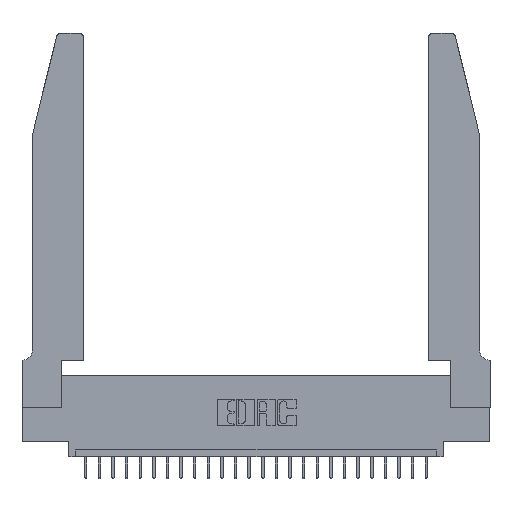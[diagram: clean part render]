
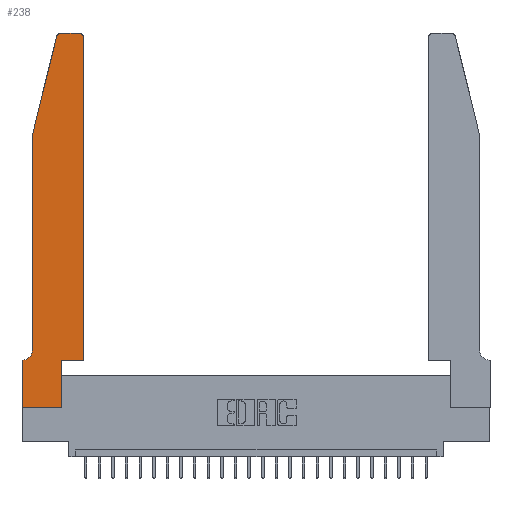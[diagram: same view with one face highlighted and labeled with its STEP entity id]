
A CAD part, top view. The second image highlights one B-rep face of the part: STEP entity #238.
In plain terms, the highlighted planar face has unit normal (0, 0, 1).
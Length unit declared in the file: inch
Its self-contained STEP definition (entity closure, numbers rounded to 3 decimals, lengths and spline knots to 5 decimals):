
#238 = ADVANCED_FACE ( 'NONE', ( #1167 ), #6195, .T. ) ;
#305 = ORIENTED_EDGE ( 'NONE', *, *, #24151, .T. ) ;
#317 = CIRCLE ( 'NONE', #17800, 0.03 ) ;
#383 = CARTESIAN_POINT ( 'NONE',  ( 0., 0., 0.37 ) ) ;
#710 = EDGE_LOOP ( 'NONE', ( #20122, #5138, #15837, #24274, #12912, #5042, #21561, #22669, #1174, #305, #4308, #14873 ) ) ;
#1167 = FACE_OUTER_BOUND ( 'NONE', #710, .T. ) ;
#1174 = ORIENTED_EDGE ( 'NONE', *, *, #11017, .T. ) ;
#1182 = LINE ( 'NONE', #8750, #21146 ) ;
#1298 = EDGE_CURVE ( 'NONE', #10869, #19458, #21773, .T. ) ;
#1369 = DIRECTION ( 'NONE',  ( 0., 1., 0. ) ) ;
#1768 = CARTESIAN_POINT ( 'NONE',  ( 0.284, 2.72, 0.37 ) ) ;
#1846 = EDGE_CURVE ( 'NONE', #4347, #19112, #21419, .T. ) ;
#1937 = EDGE_CURVE ( 'NONE', #4945, #11985, #24655, .T. ) ;
#2071 = CARTESIAN_POINT ( 'NONE',  ( 0.25487, 2.72718, 0.37 ) ) ;
#2384 = CARTESIAN_POINT ( 'NONE',  ( 0.0755, 0.42, 0.37 ) ) ;
#3088 = CARTESIAN_POINT ( 'NONE',  ( 0.4505, 0.35, 0.37 ) ) ;
#3986 = LINE ( 'NONE', #4891, #19770 ) ;
#4308 = ORIENTED_EDGE ( 'NONE', *, *, #10980, .T. ) ;
#4347 = VERTEX_POINT ( 'NONE', #4689 ) ;
#4404 = DIRECTION ( 'NONE',  ( 0., -1., 0. ) ) ;
#4645 = LINE ( 'NONE', #5413, #21703 ) ;
#4689 = CARTESIAN_POINT ( 'NONE',  ( 0., 0.35, 0.37 ) ) ;
#4891 = CARTESIAN_POINT ( 'NONE',  ( 0.2865, 0.35, 0.37 ) ) ;
#4945 = VERTEX_POINT ( 'NONE', #7746 ) ;
#5042 = ORIENTED_EDGE ( 'NONE', *, *, #24692, .T. ) ;
#5044 = CARTESIAN_POINT ( 'NONE',  ( 0.4205, 2.72, 0.37 ) ) ;
#5138 = ORIENTED_EDGE ( 'NONE', *, *, #5745, .T. ) ;
#5211 = DIRECTION ( 'NONE',  ( 1., 0., 0. ) ) ;
#5413 = CARTESIAN_POINT ( 'NONE',  ( 0.4505, 0.35, 0.37 ) ) ;
#5509 = EDGE_CURVE ( 'NONE', #13597, #10869, #10265, .T. ) ;
#5745 = EDGE_CURVE ( 'NONE', #25131, #14039, #317, .T. ) ;
#6195 = PLANE ( 'NONE',  #10839 ) ;
#6304 = LINE ( 'NONE', #13068, #21438 ) ;
#6646 = CARTESIAN_POINT ( 'NONE',  ( 0., 0.35, 0.37 ) ) ;
#6742 = DIRECTION ( 'NONE',  ( -0.239, -0.971, 0. ) ) ;
#6929 = VECTOR ( 'NONE', #10893, 39.37008 ) ;
#7746 = CARTESIAN_POINT ( 'NONE',  ( 0.4505, 2.72, 0.37 ) ) ;
#7828 = CARTESIAN_POINT ( 'NONE',  ( 0.2865, 0.35, 0.37 ) ) ;
#7952 = VECTOR ( 'NONE', #25797, 39.37008 ) ;
#8750 = CARTESIAN_POINT ( 'NONE',  ( 0.0755, 0.35, 0.37 ) ) ;
#8900 = CARTESIAN_POINT ( 'NONE',  ( 0.0755, 2., 0.37 ) ) ;
#8966 = VECTOR ( 'NONE', #4404, 39.37008 ) ;
#10160 = AXIS2_PLACEMENT_3D ( 'NONE', #5044, #19427, #5211 ) ;
#10265 = LINE ( 'NONE', #22926, #8966 ) ;
#10369 = EDGE_CURVE ( 'NONE', #11985, #25131, #21098, .T. ) ;
#10839 = AXIS2_PLACEMENT_3D ( 'NONE', #6646, #12851, #19672 ) ;
#10869 = VERTEX_POINT ( 'NONE', #2384 ) ;
#10893 = DIRECTION ( 'NONE',  ( 0., -1., 0. ) ) ;
#10980 = EDGE_CURVE ( 'NONE', #20373, #4945, #4645, .T. ) ;
#11017 = EDGE_CURVE ( 'NONE', #21164, #11185, #3986, .T. ) ;
#11185 = VERTEX_POINT ( 'NONE', #7828 ) ;
#11408 = VECTOR ( 'NONE', #14041, 39.37008 ) ;
#11512 = CARTESIAN_POINT ( 'NONE',  ( 0.0055, 0.42, 0.37 ) ) ;
#11985 = VERTEX_POINT ( 'NONE', #26577 ) ;
#12652 = CARTESIAN_POINT ( 'NONE',  ( 0.4505, 0.35, 0.37 ) ) ;
#12851 = DIRECTION ( 'NONE',  ( 0., 0., 1. ) ) ;
#12912 = ORIENTED_EDGE ( 'NONE', *, *, #1298, .T. ) ;
#13068 = CARTESIAN_POINT ( 'NONE',  ( 0., 0., 0.37 ) ) ;
#13326 = CARTESIAN_POINT ( 'NONE',  ( 0.0755, 2., 0.37 ) ) ;
#13584 = DIRECTION ( 'NONE',  ( 0., 0., -1. ) ) ;
#13597 = VERTEX_POINT ( 'NONE', #13326 ) ;
#13685 = EDGE_CURVE ( 'NONE', #19112, #21164, #6304, .T. ) ;
#13970 = LINE ( 'NONE', #8900, #21422 ) ;
#14039 = VERTEX_POINT ( 'NONE', #2071 ) ;
#14041 = DIRECTION ( 'NONE',  ( -1., 0., 0. ) ) ;
#14448 = CARTESIAN_POINT ( 'NONE',  ( 0.284, 2.75, 0.37 ) ) ;
#14873 = ORIENTED_EDGE ( 'NONE', *, *, #1937, .T. ) ;
#15837 = ORIENTED_EDGE ( 'NONE', *, *, #25254, .T. ) ;
#16302 = CARTESIAN_POINT ( 'NONE',  ( 0., 0., 0.37 ) ) ;
#16965 = LINE ( 'NONE', #3088, #7952 ) ;
#17800 = AXIS2_PLACEMENT_3D ( 'NONE', #1768, #18148, #20224 ) ;
#18148 = DIRECTION ( 'NONE',  ( 0., 0., 1. ) ) ;
#18190 = CARTESIAN_POINT ( 'NONE',  ( 0.2865, 0., 0.37 ) ) ;
#18955 = AXIS2_PLACEMENT_3D ( 'NONE', #11512, #13584, #25857 ) ;
#19112 = VERTEX_POINT ( 'NONE', #16302 ) ;
#19427 = DIRECTION ( 'NONE',  ( 0., 0., 1. ) ) ;
#19458 = VERTEX_POINT ( 'NONE', #21430 ) ;
#19672 = DIRECTION ( 'NONE',  ( 1., 0., 0. ) ) ;
#19770 = VECTOR ( 'NONE', #25956, 39.37008 ) ;
#20122 = ORIENTED_EDGE ( 'NONE', *, *, #10369, .T. ) ;
#20224 = DIRECTION ( 'NONE',  ( 1., 0., 0. ) ) ;
#20373 = VERTEX_POINT ( 'NONE', #12652 ) ;
#21098 = LINE ( 'NONE', #24153, #11408 ) ;
#21146 = VECTOR ( 'NONE', #21188, 39.37008 ) ;
#21164 = VERTEX_POINT ( 'NONE', #18190 ) ;
#21188 = DIRECTION ( 'NONE',  ( -1., 0., 0. ) ) ;
#21419 = LINE ( 'NONE', #383, #6929 ) ;
#21422 = VECTOR ( 'NONE', #6742, 39.37008 ) ;
#21430 = CARTESIAN_POINT ( 'NONE',  ( 0.0055, 0.35, 0.37 ) ) ;
#21438 = VECTOR ( 'NONE', #23505, 39.37008 ) ;
#21561 = ORIENTED_EDGE ( 'NONE', *, *, #1846, .T. ) ;
#21703 = VECTOR ( 'NONE', #1369, 39.37008 ) ;
#21773 = CIRCLE ( 'NONE', #18955, 0.07 ) ;
#22669 = ORIENTED_EDGE ( 'NONE', *, *, #13685, .T. ) ;
#22926 = CARTESIAN_POINT ( 'NONE',  ( 0.0755, 2., 0.37 ) ) ;
#23505 = DIRECTION ( 'NONE',  ( 1., 0., 0. ) ) ;
#24151 = EDGE_CURVE ( 'NONE', #11185, #20373, #16965, .T. ) ;
#24153 = CARTESIAN_POINT ( 'NONE',  ( 0.2605, 2.75, 0.37 ) ) ;
#24274 = ORIENTED_EDGE ( 'NONE', *, *, #5509, .T. ) ;
#24655 = CIRCLE ( 'NONE', #10160, 0.03 ) ;
#24692 = EDGE_CURVE ( 'NONE', #19458, #4347, #1182, .T. ) ;
#25131 = VERTEX_POINT ( 'NONE', #14448 ) ;
#25254 = EDGE_CURVE ( 'NONE', #14039, #13597, #13970, .T. ) ;
#25797 = DIRECTION ( 'NONE',  ( 1., 0., 0. ) ) ;
#25857 = DIRECTION ( 'NONE',  ( -1., 0., 0. ) ) ;
#25956 = DIRECTION ( 'NONE',  ( 0., 1., 0. ) ) ;
#26577 = CARTESIAN_POINT ( 'NONE',  ( 0.4205, 2.75, 0.37 ) ) ;
